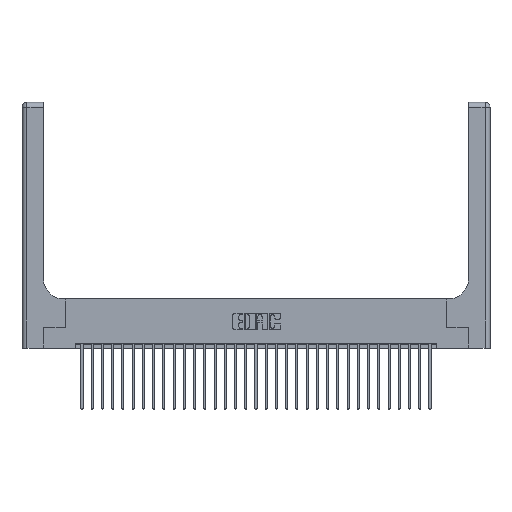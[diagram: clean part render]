
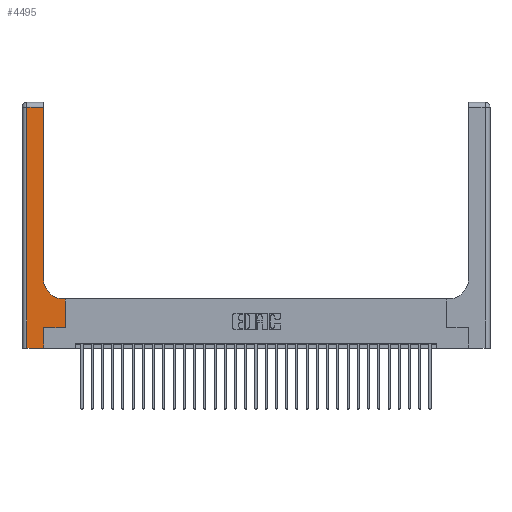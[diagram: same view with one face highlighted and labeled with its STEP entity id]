
A CAD part, top view. The second image highlights one B-rep face of the part: STEP entity #4495.
In plain terms, the highlighted planar face has unit normal (0, 0, 1).
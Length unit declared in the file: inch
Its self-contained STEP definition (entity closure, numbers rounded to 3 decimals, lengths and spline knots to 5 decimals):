
#41 = CARTESIAN_POINT ( 'NONE',  ( 0.51, 0.85, 0.37 ) ) ;
#161 = VECTOR ( 'NONE', #15271, 39.37008 ) ;
#282 = VECTOR ( 'NONE', #650, 39.37008 ) ;
#389 = CARTESIAN_POINT ( 'NONE',  ( 0., 2.94, 0.37 ) ) ;
#650 = DIRECTION ( 'NONE',  ( 0., 1., 0. ) ) ;
#1081 = CARTESIAN_POINT ( 'NONE',  ( 0.06, 2.94, 0.37 ) ) ;
#1690 = DIRECTION ( 'NONE',  ( 0., 0., -1. ) ) ;
#1800 = ORIENTED_EDGE ( 'NONE', *, *, #25017, .T. ) ;
#1903 = VERTEX_POINT ( 'NONE', #21567 ) ;
#2388 = EDGE_CURVE ( 'NONE', #28475, #24561, #10839, .T. ) ;
#2691 = ORIENTED_EDGE ( 'NONE', *, *, #6783, .T. ) ;
#4003 = VECTOR ( 'NONE', #28904, 39.37008 ) ;
#4307 = CARTESIAN_POINT ( 'NONE',  ( 0.265, 0., 0.37 ) ) ;
#4495 = ADVANCED_FACE ( 'NONE', ( #13364 ), #10817, .F. ) ;
#5102 = VERTEX_POINT ( 'NONE', #13100 ) ;
#5176 = LINE ( 'NONE', #17533, #20088 ) ;
#5746 = ORIENTED_EDGE ( 'NONE', *, *, #9153, .T. ) ;
#6783 = EDGE_CURVE ( 'NONE', #27831, #17387, #5176, .T. ) ;
#7465 = VECTOR ( 'NONE', #22784, 39.37008 ) ;
#7525 = LINE ( 'NONE', #28079, #282 ) ;
#7737 = VERTEX_POINT ( 'NONE', #9884 ) ;
#8700 = VERTEX_POINT ( 'NONE', #22116 ) ;
#8706 = DIRECTION ( 'NONE',  ( -1., 0., 0. ) ) ;
#9153 = EDGE_CURVE ( 'NONE', #12406, #28475, #26801, .T. ) ;
#9216 = CARTESIAN_POINT ( 'NONE',  ( 0.06, 0., 0.37 ) ) ;
#9359 = ORIENTED_EDGE ( 'NONE', *, *, #15434, .T. ) ;
#9643 = AXIS2_PLACEMENT_3D ( 'NONE', #29114, #1690, #8706 ) ;
#9884 = CARTESIAN_POINT ( 'NONE',  ( 0.51, 0.6, 0.37 ) ) ;
#10617 = EDGE_CURVE ( 'NONE', #7737, #8700, #28778, .T. ) ;
#10810 = EDGE_CURVE ( 'NONE', #17387, #5102, #16888, .T. ) ;
#10817 = PLANE ( 'NONE',  #9643 ) ;
#10839 = LINE ( 'NONE', #19919, #20181 ) ;
#11087 = DIRECTION ( 'NONE',  ( 1., 0., 0. ) ) ;
#11587 = LINE ( 'NONE', #389, #12686 ) ;
#12406 = VERTEX_POINT ( 'NONE', #1081 ) ;
#12686 = VECTOR ( 'NONE', #14151, 39.37008 ) ;
#13100 = CARTESIAN_POINT ( 'NONE',  ( 0.528, 0.6, 0.37 ) ) ;
#13364 = FACE_OUTER_BOUND ( 'NONE', #27845, .T. ) ;
#13496 = DIRECTION ( 'NONE',  ( 0., 0., -1. ) ) ;
#14151 = DIRECTION ( 'NONE',  ( -1., 0., 0. ) ) ;
#14307 = CARTESIAN_POINT ( 'NONE',  ( 0.528, 0.25, 0.37 ) ) ;
#14413 = CARTESIAN_POINT ( 'NONE',  ( 0.265, 0.25, 0.37 ) ) ;
#14549 = CARTESIAN_POINT ( 'NONE',  ( 0.26, 0.6, 0.37 ) ) ;
#15043 = DIRECTION ( 'NONE',  ( 1., 0., 0. ) ) ;
#15271 = DIRECTION ( 'NONE',  ( 0., -1., 0. ) ) ;
#15434 = EDGE_CURVE ( 'NONE', #5102, #7737, #19270, .T. ) ;
#15962 = AXIS2_PLACEMENT_3D ( 'NONE', #41, #13496, #11087 ) ;
#16411 = CARTESIAN_POINT ( 'NONE',  ( 0.265, 0., 0.37 ) ) ;
#16888 = LINE ( 'NONE', #28182, #4003 ) ;
#17387 = VERTEX_POINT ( 'NONE', #14307 ) ;
#17533 = CARTESIAN_POINT ( 'NONE',  ( 0.265, 0.25, 0.37 ) ) ;
#19270 = LINE ( 'NONE', #14549, #25826 ) ;
#19919 = CARTESIAN_POINT ( 'NONE',  ( 0., 0., 0.37 ) ) ;
#20088 = VECTOR ( 'NONE', #28837, 39.37008 ) ;
#20181 = VECTOR ( 'NONE', #15043, 39.37008 ) ;
#20881 = ORIENTED_EDGE ( 'NONE', *, *, #2388, .T. ) ;
#21567 = CARTESIAN_POINT ( 'NONE',  ( 0.26, 2.94, 0.37 ) ) ;
#22116 = CARTESIAN_POINT ( 'NONE',  ( 0.26, 0.85, 0.37 ) ) ;
#22675 = ORIENTED_EDGE ( 'NONE', *, *, #10617, .T. ) ;
#22784 = DIRECTION ( 'NONE',  ( 0., 1., 0. ) ) ;
#23389 = DIRECTION ( 'NONE',  ( -1., 0., 0. ) ) ;
#23937 = ORIENTED_EDGE ( 'NONE', *, *, #27776, .T. ) ;
#24561 = VERTEX_POINT ( 'NONE', #16411 ) ;
#24574 = CARTESIAN_POINT ( 'NONE',  ( 0.06, 3., 0.37 ) ) ;
#24725 = LINE ( 'NONE', #4307, #7465 ) ;
#25017 = EDGE_CURVE ( 'NONE', #1903, #12406, #11587, .T. ) ;
#25826 = VECTOR ( 'NONE', #23389, 39.37008 ) ;
#26801 = LINE ( 'NONE', #24574, #161 ) ;
#27136 = ORIENTED_EDGE ( 'NONE', *, *, #10810, .T. ) ;
#27776 = EDGE_CURVE ( 'NONE', #8700, #1903, #7525, .T. ) ;
#27831 = VERTEX_POINT ( 'NONE', #14413 ) ;
#27845 = EDGE_LOOP ( 'NONE', ( #23937, #1800, #5746, #20881, #28378, #2691, #27136, #9359, #22675 ) ) ;
#28079 = CARTESIAN_POINT ( 'NONE',  ( 0.26, 3., 0.37 ) ) ;
#28182 = CARTESIAN_POINT ( 'NONE',  ( 0.528, 0.25, 0.37 ) ) ;
#28378 = ORIENTED_EDGE ( 'NONE', *, *, #29267, .T. ) ;
#28475 = VERTEX_POINT ( 'NONE', #9216 ) ;
#28778 = CIRCLE ( 'NONE', #15962, 0.25 ) ;
#28837 = DIRECTION ( 'NONE',  ( 1., 0., 0. ) ) ;
#28904 = DIRECTION ( 'NONE',  ( 0., 1., 0. ) ) ;
#29114 = CARTESIAN_POINT ( 'NONE',  ( 0., 3., 0.37 ) ) ;
#29267 = EDGE_CURVE ( 'NONE', #24561, #27831, #24725, .T. ) ;
